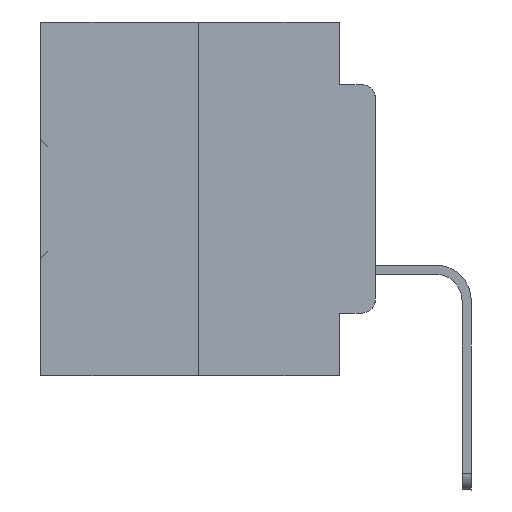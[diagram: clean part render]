
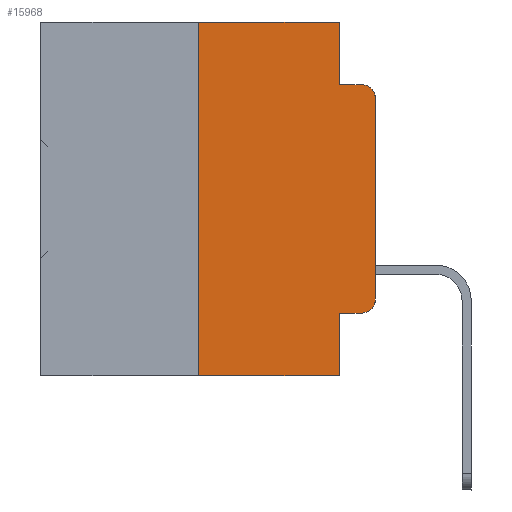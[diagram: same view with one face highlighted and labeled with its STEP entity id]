
A CAD part, left-side view. The second image highlights one B-rep face of the part: STEP entity #15968.
In plain terms, the highlighted planar face has unit normal (-1, 0, 0).
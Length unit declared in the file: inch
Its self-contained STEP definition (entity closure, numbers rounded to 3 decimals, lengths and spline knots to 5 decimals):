
#146 = CIRCLE ( 'NONE', #19397, 0.02 ) ;
#422 = DIRECTION ( 'NONE',  ( -1., 0., 0. ) ) ;
#557 = LINE ( 'NONE', #20279, #37302 ) ;
#753 = CARTESIAN_POINT ( 'NONE',  ( 0., 0.02, -0.4115 ) ) ;
#1262 = EDGE_CURVE ( 'NONE', #18506, #16109, #5101, .T. ) ;
#1932 = DIRECTION ( 'NONE',  ( 0., 0., -1. ) ) ;
#2283 = CARTESIAN_POINT ( 'NONE',  ( 0., 0.25, -0.5 ) ) ;
#2558 = VERTEX_POINT ( 'NONE', #30913 ) ;
#3107 = EDGE_CURVE ( 'NONE', #35259, #5393, #36316, .T. ) ;
#3186 = CARTESIAN_POINT ( 'NONE',  ( 0., 0.473, 0. ) ) ;
#3980 = LINE ( 'NONE', #28836, #26156 ) ;
#4360 = VECTOR ( 'NONE', #25987, 39.37008 ) ;
#4554 = CARTESIAN_POINT ( 'NONE',  ( 0., 0.473, -0.5 ) ) ;
#5101 = LINE ( 'NONE', #35225, #30918 ) ;
#5300 = ORIENTED_EDGE ( 'NONE', *, *, #1262, .T. ) ;
#5393 = VERTEX_POINT ( 'NONE', #27214 ) ;
#7650 = DIRECTION ( 'NONE',  ( -1., 0., 0. ) ) ;
#7966 = CIRCLE ( 'NONE', #16444, 0.02 ) ;
#8148 = FACE_OUTER_BOUND ( 'NONE', #20071, .T. ) ;
#8177 = EDGE_CURVE ( 'NONE', #34217, #27899, #3980, .T. ) ;
#8890 = PLANE ( 'NONE',  #18019 ) ;
#9222 = EDGE_CURVE ( 'NONE', #34266, #31541, #7966, .T. ) ;
#11568 = DIRECTION ( 'NONE',  ( 1., 0., 0. ) ) ;
#12348 = CARTESIAN_POINT ( 'NONE',  ( 0., 0.02, -0.0885 ) ) ;
#12358 = CARTESIAN_POINT ( 'NONE',  ( 0., 0., 0. ) ) ;
#12760 = DIRECTION ( 'NONE',  ( 0., 0., -1. ) ) ;
#13192 = LINE ( 'NONE', #24232, #25830 ) ;
#13356 = ORIENTED_EDGE ( 'NONE', *, *, #14161, .F. ) ;
#14161 = EDGE_CURVE ( 'NONE', #35259, #34217, #557, .T. ) ;
#14245 = VERTEX_POINT ( 'NONE', #15349 ) ;
#14804 = ORIENTED_EDGE ( 'NONE', *, *, #8177, .F. ) ;
#14924 = EDGE_CURVE ( 'NONE', #18506, #5393, #13192, .T. ) ;
#15349 = CARTESIAN_POINT ( 'NONE',  ( 0., 0., -0.3915 ) ) ;
#15411 = CARTESIAN_POINT ( 'NONE',  ( 0., 0., -0.1085 ) ) ;
#15576 = CARTESIAN_POINT ( 'NONE',  ( 0., 0.051, 0. ) ) ;
#15751 = ORIENTED_EDGE ( 'NONE', *, *, #23908, .T. ) ;
#15968 = ADVANCED_FACE ( 'NONE', ( #8148 ), #8890, .F. ) ;
#16109 = VERTEX_POINT ( 'NONE', #753 ) ;
#16375 = ORIENTED_EDGE ( 'NONE', *, *, #18310, .F. ) ;
#16444 = AXIS2_PLACEMENT_3D ( 'NONE', #30808, #7650, #1932 ) ;
#17229 = DIRECTION ( 'NONE',  ( 0., -1., 0. ) ) ;
#17548 = ORIENTED_EDGE ( 'NONE', *, *, #26392, .F. ) ;
#17795 = ORIENTED_EDGE ( 'NONE', *, *, #3107, .T. ) ;
#18019 = AXIS2_PLACEMENT_3D ( 'NONE', #3186, #11568, #31807 ) ;
#18310 = EDGE_CURVE ( 'NONE', #2558, #31541, #24693, .T. ) ;
#18506 = VERTEX_POINT ( 'NONE', #18915 ) ;
#18915 = CARTESIAN_POINT ( 'NONE',  ( 0., 0.051, -0.4115 ) ) ;
#19397 = AXIS2_PLACEMENT_3D ( 'NONE', #26492, #422, #23797 ) ;
#20071 = EDGE_LOOP ( 'NONE', ( #34361, #28220, #16375, #17548, #14804, #13356, #17795, #36015, #5300, #15751 ) ) ;
#20089 = EDGE_CURVE ( 'NONE', #14245, #34266, #31224, .T. ) ;
#20279 = CARTESIAN_POINT ( 'NONE',  ( 0., 0.25, 0. ) ) ;
#20354 = VECTOR ( 'NONE', #27271, 39.37008 ) ;
#20473 = VECTOR ( 'NONE', #36342, 39.37008 ) ;
#20526 = DIRECTION ( 'NONE',  ( 0., -1., 0. ) ) ;
#23797 = DIRECTION ( 'NONE',  ( 0., 0., -1. ) ) ;
#23908 = EDGE_CURVE ( 'NONE', #16109, #14245, #146, .T. ) ;
#24232 = CARTESIAN_POINT ( 'NONE',  ( 0., 0.051, 0. ) ) ;
#24693 = LINE ( 'NONE', #32203, #4360 ) ;
#24761 = DIRECTION ( 'NONE',  ( 0., -1., 0. ) ) ;
#25830 = VECTOR ( 'NONE', #12760, 39.37008 ) ;
#25987 = DIRECTION ( 'NONE',  ( 0., -1., 0. ) ) ;
#26141 = CARTESIAN_POINT ( 'NONE',  ( 0., 0.25, 0. ) ) ;
#26156 = VECTOR ( 'NONE', #17229, 39.37008 ) ;
#26336 = DIRECTION ( 'NONE',  ( 0., 0., 1. ) ) ;
#26392 = EDGE_CURVE ( 'NONE', #27899, #2558, #36820, .T. ) ;
#26492 = CARTESIAN_POINT ( 'NONE',  ( 0., 0.02, -0.3915 ) ) ;
#27214 = CARTESIAN_POINT ( 'NONE',  ( 0., 0.051, -0.5 ) ) ;
#27271 = DIRECTION ( 'NONE',  ( 0., 0., 1. ) ) ;
#27411 = CARTESIAN_POINT ( 'NONE',  ( 0., 0.051, 0. ) ) ;
#27899 = VERTEX_POINT ( 'NONE', #15576 ) ;
#28220 = ORIENTED_EDGE ( 'NONE', *, *, #9222, .T. ) ;
#28836 = CARTESIAN_POINT ( 'NONE',  ( 0., 0.473, 0. ) ) ;
#30808 = CARTESIAN_POINT ( 'NONE',  ( 0., 0.02, -0.1085 ) ) ;
#30913 = CARTESIAN_POINT ( 'NONE',  ( 0., 0.051, -0.0885 ) ) ;
#30918 = VECTOR ( 'NONE', #20526, 39.37008 ) ;
#31224 = LINE ( 'NONE', #12358, #20354 ) ;
#31541 = VERTEX_POINT ( 'NONE', #12348 ) ;
#31807 = DIRECTION ( 'NONE',  ( 0., 0., -1. ) ) ;
#32203 = CARTESIAN_POINT ( 'NONE',  ( 0., 0.051, -0.0885 ) ) ;
#34217 = VERTEX_POINT ( 'NONE', #26141 ) ;
#34266 = VERTEX_POINT ( 'NONE', #15411 ) ;
#34361 = ORIENTED_EDGE ( 'NONE', *, *, #20089, .T. ) ;
#35225 = CARTESIAN_POINT ( 'NONE',  ( 0., 0.051, -0.4115 ) ) ;
#35259 = VERTEX_POINT ( 'NONE', #2283 ) ;
#35381 = VECTOR ( 'NONE', #24761, 39.37008 ) ;
#36015 = ORIENTED_EDGE ( 'NONE', *, *, #14924, .F. ) ;
#36316 = LINE ( 'NONE', #4554, #35381 ) ;
#36342 = DIRECTION ( 'NONE',  ( 0., 0., -1. ) ) ;
#36820 = LINE ( 'NONE', #27411, #20473 ) ;
#37302 = VECTOR ( 'NONE', #26336, 39.37008 ) ;
